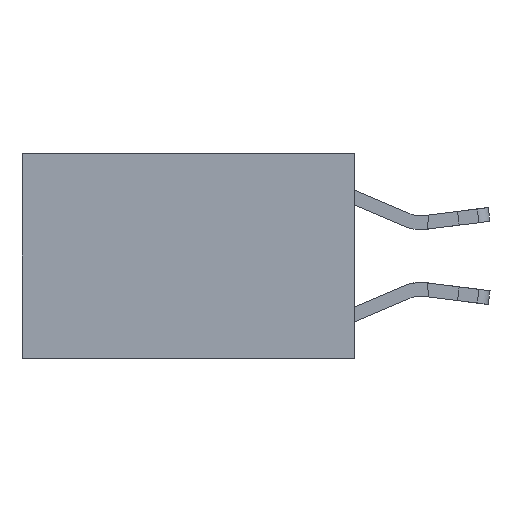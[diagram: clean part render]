
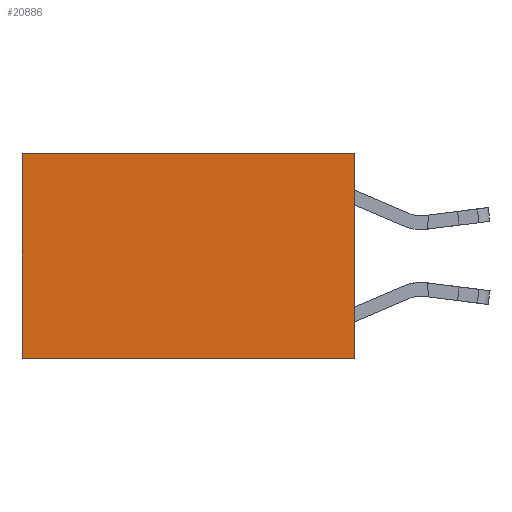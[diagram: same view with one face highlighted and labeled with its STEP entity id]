
A CAD part, left-side view. The second image highlights one B-rep face of the part: STEP entity #20886.
In plain terms, the highlighted planar face has unit normal (-1, 0, 0).
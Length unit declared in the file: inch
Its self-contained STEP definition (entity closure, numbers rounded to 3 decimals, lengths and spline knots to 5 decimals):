
#173 = DIRECTION ( 'NONE',  ( 1., 0., 0. ) ) ;
#1309 = EDGE_LOOP ( 'NONE', ( #9879, #11444, #19204, #11061 ) ) ;
#2925 = CARTESIAN_POINT ( 'NONE',  ( 0.2625, 0.6, 0. ) ) ;
#3901 = VECTOR ( 'NONE', #17936, 39.37008 ) ;
#3955 = VECTOR ( 'NONE', #22934, 39.37008 ) ;
#4862 = CARTESIAN_POINT ( 'NONE',  ( 0.2625, 0.6, 0. ) ) ;
#4966 = EDGE_CURVE ( 'NONE', #17469, #17819, #19206, .T. ) ;
#5082 = EDGE_CURVE ( 'NONE', #17059, #17819, #19046, .T. ) ;
#5198 = LINE ( 'NONE', #21681, #14791 ) ;
#6708 = EDGE_CURVE ( 'NONE', #9625, #17469, #8434, .T. ) ;
#6816 = DIRECTION ( 'NONE',  ( 0., 0., -1. ) ) ;
#7391 = CARTESIAN_POINT ( 'NONE',  ( 0.2625, 0., 0. ) ) ;
#8434 = LINE ( 'NONE', #9493, #3955 ) ;
#8643 = CARTESIAN_POINT ( 'NONE',  ( 0.2625, 0.6, -0.37 ) ) ;
#9493 = CARTESIAN_POINT ( 'NONE',  ( 0.2625, 0., 0. ) ) ;
#9578 = AXIS2_PLACEMENT_3D ( 'NONE', #11684, #173, #13641 ) ;
#9625 = VERTEX_POINT ( 'NONE', #7391 ) ;
#9690 = CARTESIAN_POINT ( 'NONE',  ( 0.2625, 0., -0.37 ) ) ;
#9879 = ORIENTED_EDGE ( 'NONE', *, *, #5082, .T. ) ;
#11061 = ORIENTED_EDGE ( 'NONE', *, *, #12068, .T. ) ;
#11404 = FACE_OUTER_BOUND ( 'NONE', #1309, .T. ) ;
#11444 = ORIENTED_EDGE ( 'NONE', *, *, #4966, .F. ) ;
#11684 = CARTESIAN_POINT ( 'NONE',  ( 0.2625, 0., 0. ) ) ;
#12068 = EDGE_CURVE ( 'NONE', #9625, #17059, #5198, .T. ) ;
#12154 = CARTESIAN_POINT ( 'NONE',  ( 0.2625, 0., -0.37 ) ) ;
#13641 = DIRECTION ( 'NONE',  ( 0., 0., -1. ) ) ;
#14791 = VECTOR ( 'NONE', #23631, 39.37008 ) ;
#17059 = VERTEX_POINT ( 'NONE', #2925 ) ;
#17469 = VERTEX_POINT ( 'NONE', #9690 ) ;
#17819 = VERTEX_POINT ( 'NONE', #8643 ) ;
#17936 = DIRECTION ( 'NONE',  ( 0., 1., 0. ) ) ;
#18436 = VECTOR ( 'NONE', #6816, 39.37008 ) ;
#19046 = LINE ( 'NONE', #4862, #18436 ) ;
#19204 = ORIENTED_EDGE ( 'NONE', *, *, #6708, .F. ) ;
#19206 = LINE ( 'NONE', #12154, #3901 ) ;
#20886 = ADVANCED_FACE ( 'NONE', ( #11404 ), #23197, .F. ) ;
#21681 = CARTESIAN_POINT ( 'NONE',  ( 0.2625, 0., 0. ) ) ;
#22934 = DIRECTION ( 'NONE',  ( 0., 0., -1. ) ) ;
#23197 = PLANE ( 'NONE',  #9578 ) ;
#23631 = DIRECTION ( 'NONE',  ( 0., 1., 0. ) ) ;
